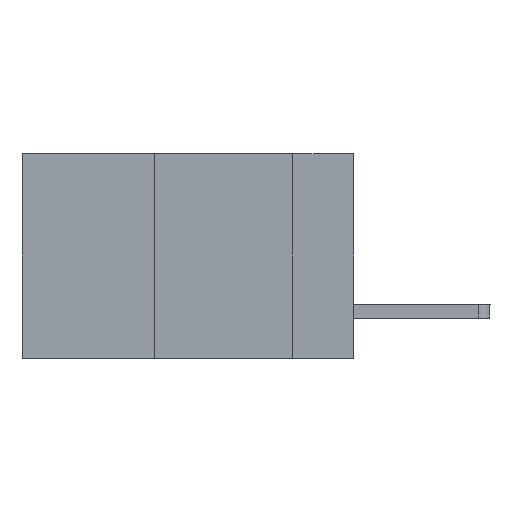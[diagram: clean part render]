
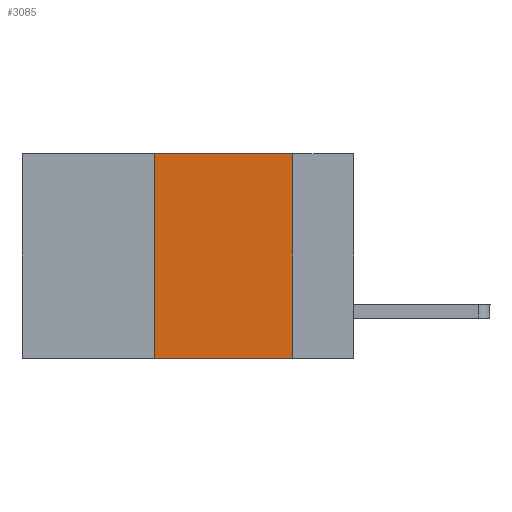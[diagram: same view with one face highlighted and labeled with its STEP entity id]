
A CAD part, left-side view. The second image highlights one B-rep face of the part: STEP entity #3085.
In plain terms, the highlighted planar face has unit normal (-1, 0, 0).
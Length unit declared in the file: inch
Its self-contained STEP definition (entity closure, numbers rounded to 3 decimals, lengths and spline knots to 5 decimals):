
#162 = VECTOR ( 'NONE', #8858, 39.37008 ) ;
#734 = CARTESIAN_POINT ( 'NONE',  ( 0., 0.6, 0. ) ) ;
#1382 = CARTESIAN_POINT ( 'NONE',  ( 0., 0.11, -0.37 ) ) ;
#2225 = EDGE_CURVE ( 'NONE', #3155, #9806, #8742, .T. ) ;
#2824 = DIRECTION ( 'NONE',  ( 1., 0., 0. ) ) ;
#3085 = ADVANCED_FACE ( 'NONE', ( #10225 ), #7543, .F. ) ;
#3095 = CARTESIAN_POINT ( 'NONE',  ( 0., 0.36, 0. ) ) ;
#3155 = VERTEX_POINT ( 'NONE', #5881 ) ;
#3652 = EDGE_CURVE ( 'NONE', #5335, #7971, #10209, .T. ) ;
#3680 = DIRECTION ( 'NONE',  ( 0., 0., -1. ) ) ;
#4185 = LINE ( 'NONE', #6324, #7299 ) ;
#4240 = VECTOR ( 'NONE', #6408, 39.37008 ) ;
#4528 = CARTESIAN_POINT ( 'NONE',  ( 0., 0.11, 0. ) ) ;
#4543 = LINE ( 'NONE', #734, #4240 ) ;
#4692 = CARTESIAN_POINT ( 'NONE',  ( 0., 0.6, 0. ) ) ;
#4967 = VECTOR ( 'NONE', #9553, 39.37008 ) ;
#5185 = ORIENTED_EDGE ( 'NONE', *, *, #2225, .F. ) ;
#5335 = VERTEX_POINT ( 'NONE', #4528 ) ;
#5881 = CARTESIAN_POINT ( 'NONE',  ( 0., 0.36, -0.37 ) ) ;
#6324 = CARTESIAN_POINT ( 'NONE',  ( 0., 0.6, -0.37 ) ) ;
#6408 = DIRECTION ( 'NONE',  ( 0., -1., 0. ) ) ;
#6693 = ORIENTED_EDGE ( 'NONE', *, *, #3652, .F. ) ;
#7299 = VECTOR ( 'NONE', #10016, 39.37008 ) ;
#7543 = PLANE ( 'NONE',  #8104 ) ;
#7562 = ORIENTED_EDGE ( 'NONE', *, *, #8733, .F. ) ;
#7971 = VERTEX_POINT ( 'NONE', #1382 ) ;
#8104 = AXIS2_PLACEMENT_3D ( 'NONE', #4692, #2824, #3680 ) ;
#8586 = CARTESIAN_POINT ( 'NONE',  ( 0., 0.11, 0. ) ) ;
#8733 = EDGE_CURVE ( 'NONE', #9806, #5335, #4543, .T. ) ;
#8742 = LINE ( 'NONE', #3095, #162 ) ;
#8858 = DIRECTION ( 'NONE',  ( 0., 0., 1. ) ) ;
#9553 = DIRECTION ( 'NONE',  ( 0., 0., -1. ) ) ;
#9806 = VERTEX_POINT ( 'NONE', #11510 ) ;
#10016 = DIRECTION ( 'NONE',  ( 0., -1., 0. ) ) ;
#10209 = LINE ( 'NONE', #8586, #4967 ) ;
#10225 = FACE_OUTER_BOUND ( 'NONE', #12023, .T. ) ;
#10628 = EDGE_CURVE ( 'NONE', #3155, #7971, #4185, .T. ) ;
#11336 = ORIENTED_EDGE ( 'NONE', *, *, #10628, .T. ) ;
#11510 = CARTESIAN_POINT ( 'NONE',  ( 0., 0.36, 0. ) ) ;
#12023 = EDGE_LOOP ( 'NONE', ( #6693, #7562, #5185, #11336 ) ) ;
